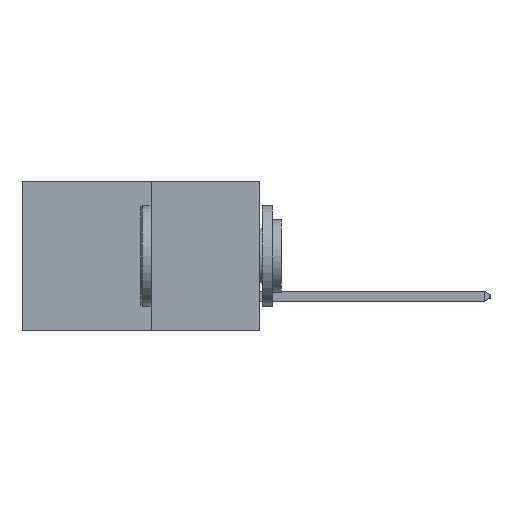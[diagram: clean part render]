
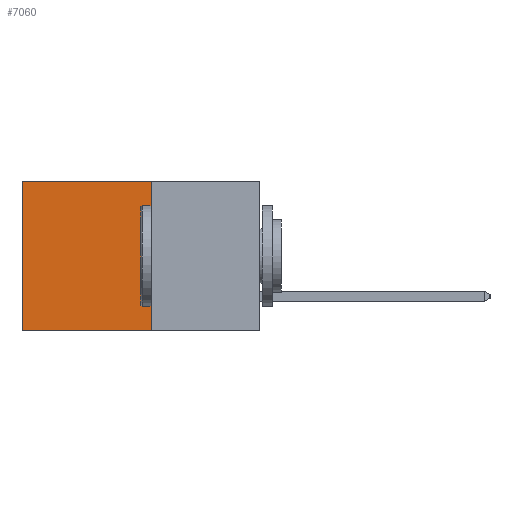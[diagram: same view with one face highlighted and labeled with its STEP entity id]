
A CAD part, left-side view. The second image highlights one B-rep face of the part: STEP entity #7060.
In plain terms, the highlighted planar face has unit normal (-1, 0, 0).
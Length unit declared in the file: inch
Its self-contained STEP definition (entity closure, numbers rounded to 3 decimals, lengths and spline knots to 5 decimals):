
#94 = EDGE_CURVE ( 'NONE', #7290, #7193, #1348, .T. ) ;
#403 = CARTESIAN_POINT ( 'NONE',  ( 0.277, 0.27, -0.37 ) ) ;
#696 = CARTESIAN_POINT ( 'NONE',  ( 0.277, 0.59, 0. ) ) ;
#845 = DIRECTION ( 'NONE',  ( 0., 0., -1. ) ) ;
#854 = DIRECTION ( 'NONE',  ( 1., 0., 0. ) ) ;
#908 = CARTESIAN_POINT ( 'NONE',  ( 0.277, 0.27, -0.37 ) ) ;
#929 = PLANE ( 'NONE',  #9789 ) ;
#1348 = LINE ( 'NONE', #10264, #7527 ) ;
#1657 = CARTESIAN_POINT ( 'NONE',  ( 0.277, 0.27, 0. ) ) ;
#1699 = DIRECTION ( 'NONE',  ( 0., 1., 0. ) ) ;
#1799 = VERTEX_POINT ( 'NONE', #4312 ) ;
#1994 = LINE ( 'NONE', #2079, #9793 ) ;
#2079 = CARTESIAN_POINT ( 'NONE',  ( 0.277, 0.27, -0.37 ) ) ;
#2233 = EDGE_CURVE ( 'NONE', #1799, #7106, #4341, .T. ) ;
#2811 = ORIENTED_EDGE ( 'NONE', *, *, #6100, .T. ) ;
#2859 = ORIENTED_EDGE ( 'NONE', *, *, #94, .F. ) ;
#2892 = ORIENTED_EDGE ( 'NONE', *, *, #9279, .F. ) ;
#2913 = ORIENTED_EDGE ( 'NONE', *, *, #2233, .T. ) ;
#2985 = DIRECTION ( 'NONE',  ( 0., 0., -1. ) ) ;
#3106 = EDGE_LOOP ( 'NONE', ( #2811, #2859, #2892, #2913 ) ) ;
#3553 = LINE ( 'NONE', #7620, #7890 ) ;
#4312 = CARTESIAN_POINT ( 'NONE',  ( 0.277, 0.27, 0. ) ) ;
#4341 = LINE ( 'NONE', #1657, #5916 ) ;
#5916 = VECTOR ( 'NONE', #1699, 39.37008 ) ;
#6100 = EDGE_CURVE ( 'NONE', #7106, #7193, #3553, .T. ) ;
#7060 = ADVANCED_FACE ( 'NONE', ( #8248 ), #929, .F. ) ;
#7106 = VERTEX_POINT ( 'NONE', #696 ) ;
#7193 = VERTEX_POINT ( 'NONE', #10274 ) ;
#7290 = VERTEX_POINT ( 'NONE', #403 ) ;
#7527 = VECTOR ( 'NONE', #9380, 39.37008 ) ;
#7595 = DIRECTION ( 'NONE',  ( 0., 0., -1. ) ) ;
#7620 = CARTESIAN_POINT ( 'NONE',  ( 0.277, 0.59, -0.37 ) ) ;
#7890 = VECTOR ( 'NONE', #7595, 39.37008 ) ;
#8248 = FACE_OUTER_BOUND ( 'NONE', #3106, .T. ) ;
#9279 = EDGE_CURVE ( 'NONE', #1799, #7290, #1994, .T. ) ;
#9380 = DIRECTION ( 'NONE',  ( 0., 1., 0. ) ) ;
#9789 = AXIS2_PLACEMENT_3D ( 'NONE', #908, #854, #845 ) ;
#9793 = VECTOR ( 'NONE', #2985, 39.37008 ) ;
#10264 = CARTESIAN_POINT ( 'NONE',  ( 0.277, 0.27, -0.37 ) ) ;
#10274 = CARTESIAN_POINT ( 'NONE',  ( 0.277, 0.59, -0.37 ) ) ;
